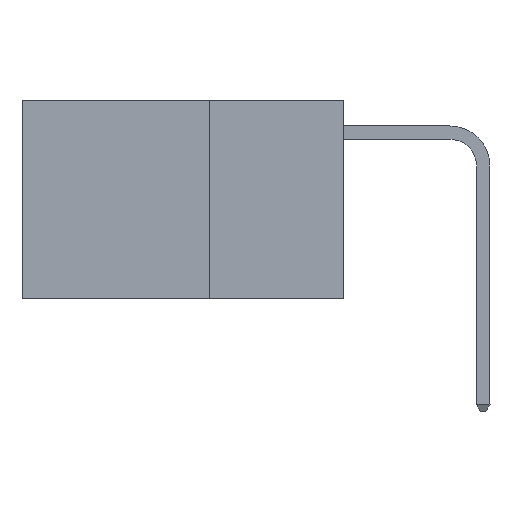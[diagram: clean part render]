
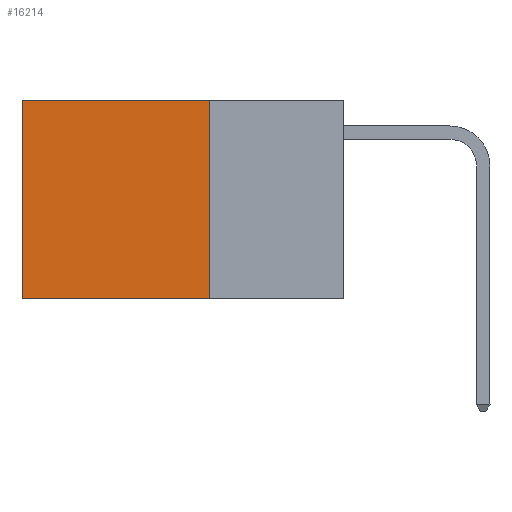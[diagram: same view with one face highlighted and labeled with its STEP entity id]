
A CAD part, left-side view. The second image highlights one B-rep face of the part: STEP entity #16214.
In plain terms, the highlighted planar face has unit normal (-1, 0, 0).
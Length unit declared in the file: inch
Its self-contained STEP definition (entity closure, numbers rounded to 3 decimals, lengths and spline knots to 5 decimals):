
#172 = LINE ( 'NONE', #20140, #7396 ) ;
#186 = DIRECTION ( 'NONE',  ( 0., 0., -1. ) ) ;
#362 = CARTESIAN_POINT ( 'NONE',  ( 0.2625, 0.25, 0. ) ) ;
#701 = VERTEX_POINT ( 'NONE', #4497 ) ;
#818 = VECTOR ( 'NONE', #9042, 39.37008 ) ;
#864 = VERTEX_POINT ( 'NONE', #23114 ) ;
#1386 = LINE ( 'NONE', #8531, #7692 ) ;
#1683 = EDGE_CURVE ( 'NONE', #4917, #864, #11655, .T. ) ;
#2437 = DIRECTION ( 'NONE',  ( 0., 1., 0. ) ) ;
#3289 = DIRECTION ( 'NONE',  ( 0., 0., -1. ) ) ;
#4497 = CARTESIAN_POINT ( 'NONE',  ( 0.2625, 0.25, -0.37 ) ) ;
#4917 = VERTEX_POINT ( 'NONE', #14280 ) ;
#6180 = VECTOR ( 'NONE', #6271, 39.37008 ) ;
#6271 = DIRECTION ( 'NONE',  ( 0., 0., -1. ) ) ;
#6304 = ORIENTED_EDGE ( 'NONE', *, *, #16290, .F. ) ;
#7396 = VECTOR ( 'NONE', #2437, 39.37008 ) ;
#7692 = VECTOR ( 'NONE', #186, 39.37008 ) ;
#8419 = ORIENTED_EDGE ( 'NONE', *, *, #1683, .T. ) ;
#8531 = CARTESIAN_POINT ( 'NONE',  ( 0.2625, 0.25, 0. ) ) ;
#9042 = DIRECTION ( 'NONE',  ( 0., 1., 0. ) ) ;
#9162 = CARTESIAN_POINT ( 'NONE',  ( 0.2625, 0.25, 0. ) ) ;
#10359 = EDGE_CURVE ( 'NONE', #15644, #4917, #19863, .T. ) ;
#11655 = LINE ( 'NONE', #22366, #6180 ) ;
#11903 = ORIENTED_EDGE ( 'NONE', *, *, #10359, .T. ) ;
#12150 = CARTESIAN_POINT ( 'NONE',  ( 0.2625, 0.25, 0. ) ) ;
#13986 = PLANE ( 'NONE',  #20458 ) ;
#14280 = CARTESIAN_POINT ( 'NONE',  ( 0.2625, 0.6, 0. ) ) ;
#15644 = VERTEX_POINT ( 'NONE', #9162 ) ;
#16214 = ADVANCED_FACE ( 'NONE', ( #21082 ), #13986, .F. ) ;
#16290 = EDGE_CURVE ( 'NONE', #15644, #701, #1386, .T. ) ;
#18136 = EDGE_LOOP ( 'NONE', ( #8419, #19514, #6304, #11903 ) ) ;
#19111 = EDGE_CURVE ( 'NONE', #701, #864, #172, .T. ) ;
#19514 = ORIENTED_EDGE ( 'NONE', *, *, #19111, .F. ) ;
#19863 = LINE ( 'NONE', #362, #818 ) ;
#20140 = CARTESIAN_POINT ( 'NONE',  ( 0.2625, 0.25, -0.37 ) ) ;
#20458 = AXIS2_PLACEMENT_3D ( 'NONE', #12150, #23070, #3289 ) ;
#21082 = FACE_OUTER_BOUND ( 'NONE', #18136, .T. ) ;
#22366 = CARTESIAN_POINT ( 'NONE',  ( 0.2625, 0.6, 0. ) ) ;
#23070 = DIRECTION ( 'NONE',  ( 1., 0., 0. ) ) ;
#23114 = CARTESIAN_POINT ( 'NONE',  ( 0.2625, 0.6, -0.37 ) ) ;
